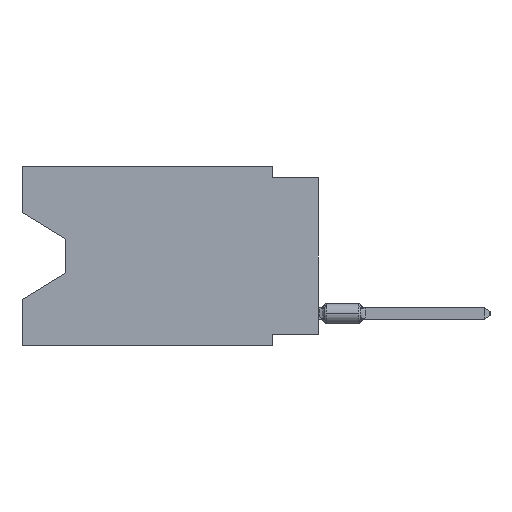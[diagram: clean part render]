
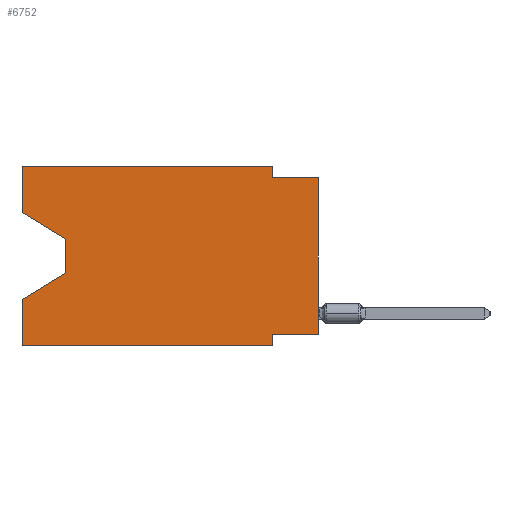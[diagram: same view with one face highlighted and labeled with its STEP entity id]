
A CAD part, left-side view. The second image highlights one B-rep face of the part: STEP entity #6752.
In plain terms, the highlighted planar face has unit normal (-1, 0, 0).
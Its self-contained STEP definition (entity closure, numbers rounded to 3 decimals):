
#192 = VECTOR ( 'NONE', #17913, 1000. ) ;
#508 = DIRECTION ( 'NONE',  ( 0., -1., 0. ) ) ;
#866 = VECTOR ( 'NONE', #17977, 1000. ) ;
#1912 = VERTEX_POINT ( 'NONE', #17825 ) ;
#2264 = LINE ( 'NONE', #22520, #17420 ) ;
#3139 = VECTOR ( 'NONE', #8559, 1000. ) ;
#3621 = EDGE_CURVE ( 'NONE', #6252, #31280, #36358, .T. ) ;
#3976 = LINE ( 'NONE', #17685, #19218 ) ;
#4269 = VECTOR ( 'NONE', #508, 1000. ) ;
#4741 = LINE ( 'NONE', #31277, #34920 ) ;
#4979 = EDGE_CURVE ( 'NONE', #28948, #20035, #3976, .T. ) ;
#5095 = VECTOR ( 'NONE', #10573, 1000. ) ;
#5470 = CARTESIAN_POINT ( 'NONE',  ( 0., 16.383, 0. ) ) ;
#6252 = VERTEX_POINT ( 'NONE', #18590 ) ;
#6589 = CARTESIAN_POINT ( 'NONE',  ( 0., 2.54, 0. ) ) ;
#6752 = ADVANCED_FACE ( 'NONE', ( #22227 ), #25702, .F. ) ;
#7458 = VERTEX_POINT ( 'NONE', #23372 ) ;
#7577 = EDGE_CURVE ( 'NONE', #35400, #23420, #31604, .T. ) ;
#7999 = ORIENTED_EDGE ( 'NONE', *, *, #25381, .T. ) ;
#8257 = ORIENTED_EDGE ( 'NONE', *, *, #14598, .T. ) ;
#8312 = CARTESIAN_POINT ( 'NONE',  ( 0., 13.97, -4.013 ) ) ;
#8559 = DIRECTION ( 'NONE',  ( 0., -1., 0. ) ) ;
#9900 = VECTOR ( 'NONE', #17133, 1000. ) ;
#10474 = EDGE_CURVE ( 'NONE', #31280, #24609, #28363, .T. ) ;
#10573 = DIRECTION ( 'NONE',  ( 0., 1., 0. ) ) ;
#11461 = CARTESIAN_POINT ( 'NONE',  ( 0., 16.383, 0. ) ) ;
#11998 = EDGE_CURVE ( 'NONE', #16762, #1912, #39873, .T. ) ;
#12014 = LINE ( 'NONE', #20808, #9900 ) ;
#12282 = CARTESIAN_POINT ( 'NONE',  ( 0., 2.54, -9.271 ) ) ;
#13184 = CARTESIAN_POINT ( 'NONE',  ( 0., 16.383, 0. ) ) ;
#13636 = VERTEX_POINT ( 'NONE', #17226 ) ;
#14077 = CARTESIAN_POINT ( 'NONE',  ( 0., 0., -0.635 ) ) ;
#14223 = VECTOR ( 'NONE', #36815, 1000. ) ;
#14598 = EDGE_CURVE ( 'NONE', #28948, #35400, #12014, .T. ) ;
#14735 = DIRECTION ( 'NONE',  ( 0., 0.855, -0.519 ) ) ;
#15367 = EDGE_CURVE ( 'NONE', #7458, #35771, #22995, .T. ) ;
#16276 = DIRECTION ( 'NONE',  ( 0., 0., 1. ) ) ;
#16762 = VERTEX_POINT ( 'NONE', #29931 ) ;
#17102 = ORIENTED_EDGE ( 'NONE', *, *, #39024, .F. ) ;
#17133 = DIRECTION ( 'NONE',  ( 0., -0.855, -0.519 ) ) ;
#17226 = CARTESIAN_POINT ( 'NONE',  ( 0., 2.54, -9.906 ) ) ;
#17420 = VECTOR ( 'NONE', #35744, 1000. ) ;
#17685 = CARTESIAN_POINT ( 'NONE',  ( 0., 16.383, 0. ) ) ;
#17825 = CARTESIAN_POINT ( 'NONE',  ( 0., 16.383, -7.36 ) ) ;
#17913 = DIRECTION ( 'NONE',  ( 0., 0., -1. ) ) ;
#17977 = DIRECTION ( 'NONE',  ( 0., -1., 0. ) ) ;
#17982 = ORIENTED_EDGE ( 'NONE', *, *, #7577, .T. ) ;
#18000 = ORIENTED_EDGE ( 'NONE', *, *, #33100, .T. ) ;
#18127 = ORIENTED_EDGE ( 'NONE', *, *, #20770, .F. ) ;
#18590 = CARTESIAN_POINT ( 'NONE',  ( 0., 2.54, 0. ) ) ;
#18628 = EDGE_LOOP ( 'NONE', ( #8257, #17982, #23291, #33872, #7999, #18127, #37247, #18000, #22083, #31811, #17102, #39042 ) ) ;
#19218 = VECTOR ( 'NONE', #37225, 1000. ) ;
#19874 = LINE ( 'NONE', #23139, #4269 ) ;
#20035 = VERTEX_POINT ( 'NONE', #11461 ) ;
#20770 = EDGE_CURVE ( 'NONE', #35771, #13636, #2264, .T. ) ;
#20808 = CARTESIAN_POINT ( 'NONE',  ( 0., 16.383, -2.546 ) ) ;
#21410 = CARTESIAN_POINT ( 'NONE',  ( 0., 13.97, -4.013 ) ) ;
#22083 = ORIENTED_EDGE ( 'NONE', *, *, #10474, .F. ) ;
#22227 = FACE_OUTER_BOUND ( 'NONE', #18628, .T. ) ;
#22520 = CARTESIAN_POINT ( 'NONE',  ( 0., 2.54, -9.906 ) ) ;
#22867 = DIRECTION ( 'NONE',  ( 0., 0., -1. ) ) ;
#22995 = LINE ( 'NONE', #26905, #5095 ) ;
#23139 = CARTESIAN_POINT ( 'NONE',  ( 0., 16.383, -9.906 ) ) ;
#23291 = ORIENTED_EDGE ( 'NONE', *, *, #23567, .T. ) ;
#23372 = CARTESIAN_POINT ( 'NONE',  ( 0., 0., -9.271 ) ) ;
#23420 = VERTEX_POINT ( 'NONE', #36494 ) ;
#23567 = EDGE_CURVE ( 'NONE', #23420, #1912, #4741, .T. ) ;
#24609 = VERTEX_POINT ( 'NONE', #14077 ) ;
#25381 = EDGE_CURVE ( 'NONE', #16762, #13636, #19874, .T. ) ;
#25604 = AXIS2_PLACEMENT_3D ( 'NONE', #5470, #35448, #22867 ) ;
#25702 = PLANE ( 'NONE',  #25604 ) ;
#26279 = CARTESIAN_POINT ( 'NONE',  ( 0., 0., 0. ) ) ;
#26905 = CARTESIAN_POINT ( 'NONE',  ( 0., 0., -9.271 ) ) ;
#28363 = LINE ( 'NONE', #41161, #3139 ) ;
#28901 = LINE ( 'NONE', #26279, #29950 ) ;
#28948 = VERTEX_POINT ( 'NONE', #42646 ) ;
#29694 = CARTESIAN_POINT ( 'NONE',  ( 0., 2.54, -0.635 ) ) ;
#29931 = CARTESIAN_POINT ( 'NONE',  ( 0., 16.383, -9.906 ) ) ;
#29950 = VECTOR ( 'NONE', #16276, 1000. ) ;
#31277 = CARTESIAN_POINT ( 'NONE',  ( 0., 13.97, -5.893 ) ) ;
#31280 = VERTEX_POINT ( 'NONE', #29694 ) ;
#31604 = LINE ( 'NONE', #8312, #192 ) ;
#31811 = ORIENTED_EDGE ( 'NONE', *, *, #3621, .F. ) ;
#33100 = EDGE_CURVE ( 'NONE', #7458, #24609, #28901, .T. ) ;
#33121 = DIRECTION ( 'NONE',  ( 0., 0., -1. ) ) ;
#33872 = ORIENTED_EDGE ( 'NONE', *, *, #11998, .F. ) ;
#34920 = VECTOR ( 'NONE', #14735, 1000. ) ;
#35400 = VERTEX_POINT ( 'NONE', #21410 ) ;
#35448 = DIRECTION ( 'NONE',  ( 1., 0., 0. ) ) ;
#35744 = DIRECTION ( 'NONE',  ( 0., 0., -1. ) ) ;
#35771 = VERTEX_POINT ( 'NONE', #12282 ) ;
#36358 = LINE ( 'NONE', #6589, #40652 ) ;
#36403 = CARTESIAN_POINT ( 'NONE',  ( 0., 16.383, 0. ) ) ;
#36494 = CARTESIAN_POINT ( 'NONE',  ( 0., 13.97, -5.893 ) ) ;
#36815 = DIRECTION ( 'NONE',  ( 0., 0., 1. ) ) ;
#37225 = DIRECTION ( 'NONE',  ( 0., 0., 1. ) ) ;
#37247 = ORIENTED_EDGE ( 'NONE', *, *, #15367, .F. ) ;
#39024 = EDGE_CURVE ( 'NONE', #20035, #6252, #42940, .T. ) ;
#39042 = ORIENTED_EDGE ( 'NONE', *, *, #4979, .F. ) ;
#39873 = LINE ( 'NONE', #36403, #14223 ) ;
#40652 = VECTOR ( 'NONE', #33121, 1000. ) ;
#41161 = CARTESIAN_POINT ( 'NONE',  ( 0., 0., -0.635 ) ) ;
#42646 = CARTESIAN_POINT ( 'NONE',  ( 0., 16.383, -2.546 ) ) ;
#42940 = LINE ( 'NONE', #13184, #866 ) ;
